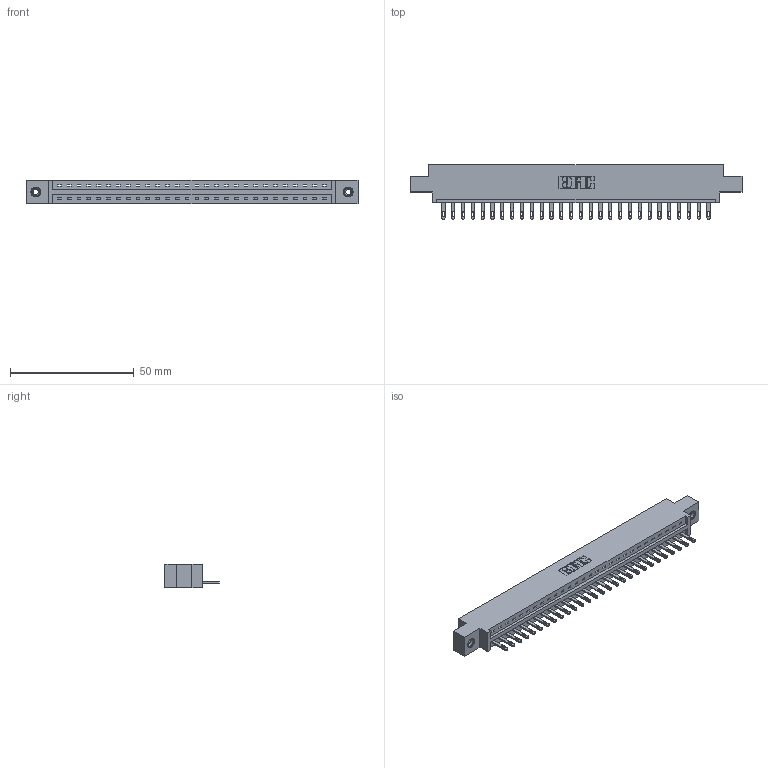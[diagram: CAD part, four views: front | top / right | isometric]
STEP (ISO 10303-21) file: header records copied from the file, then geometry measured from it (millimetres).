
FILE_DESCRIPTION (( 'STEP AP203' ), '1' );
FILE_NAME ('887-028-500-608.STEP', '2020-09-20T20:11:17', ( '' ), ( '' ), 'SwSTEP 2.0', 'SolidWorks 2020', '' );
FILE_SCHEMA (( 'CONFIG_CONTROL_DESIGN' ));
Length unit declared in the file: inch
Products named in the file (4): 345-292-001_345-293-100; 887-028-500-608; 345-250-001_345-250-003-102; 837 Part_0.170 Offset - 0.156 Dia-TI
Assembly tree (31 placements, depth 2):
  887-028-500-608
    837 Part_0.170 Offset - 0.156 Dia-TI
    345-292-001_345-293-100  x28
    345-250-001_345-250-003-102  x2
Bounding box: 133.96 x 21.85 x 9.4 mm (x, y, z)
Volume: 13641 mm3; surface area: 14209.7 mm2
Topology: 31 solids, 31 shells, 1802 faces, 5499 edges, 3658 vertices
Faces by surface type: plane 1226, cylinder 560, cone 12, torus 4
Entity records: 23872 total; most frequent: CARTESIAN_POINT 4137, ORIENTED_EDGE 4094, DIRECTION 3545, EDGE_CURVE 2047, LINE 1895, VECTOR 1895, VERTEX_POINT 1360, AXIS2_PLACEMENT_3D 825
